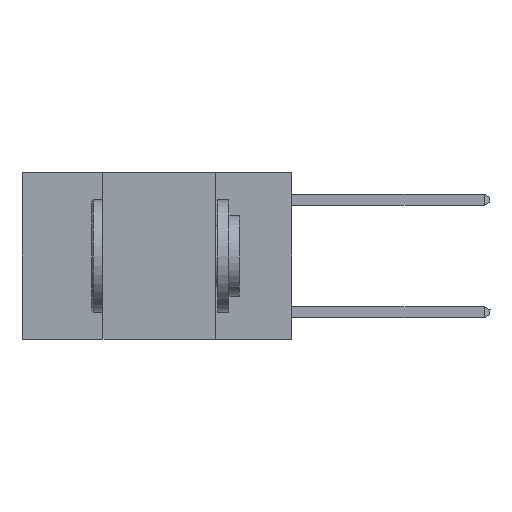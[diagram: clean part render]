
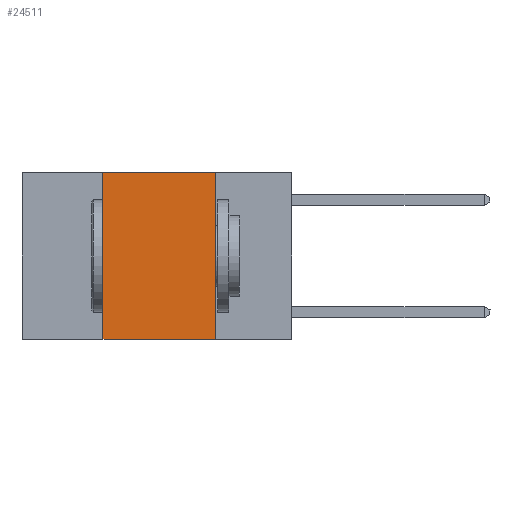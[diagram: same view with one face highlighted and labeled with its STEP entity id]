
A CAD part, left-side view. The second image highlights one B-rep face of the part: STEP entity #24511.
In plain terms, the highlighted planar face has unit normal (-1, 0, 0).
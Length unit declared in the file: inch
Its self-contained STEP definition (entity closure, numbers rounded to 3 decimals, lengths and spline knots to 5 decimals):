
#181 = DIRECTION ( 'NONE',  ( 0., -1., 0. ) ) ;
#733 = ORIENTED_EDGE ( 'NONE', *, *, #6501, .T. ) ;
#1856 = VERTEX_POINT ( 'NONE', #21726 ) ;
#4850 = VERTEX_POINT ( 'NONE', #27027 ) ;
#6138 = DIRECTION ( 'NONE',  ( 0., -1., 0. ) ) ;
#6285 = DIRECTION ( 'NONE',  ( 0., 0., 1. ) ) ;
#6501 = EDGE_CURVE ( 'NONE', #29805, #9033, #10581, .T. ) ;
#7620 = AXIS2_PLACEMENT_3D ( 'NONE', #12785, #10416, #27014 ) ;
#9033 = VERTEX_POINT ( 'NONE', #15039 ) ;
#9204 = VECTOR ( 'NONE', #28720, 39.37008 ) ;
#9432 = VECTOR ( 'NONE', #6285, 39.37008 ) ;
#10416 = DIRECTION ( 'NONE',  ( 1., 0., 0. ) ) ;
#10581 = LINE ( 'NONE', #18218, #16309 ) ;
#12785 = CARTESIAN_POINT ( 'NONE',  ( 0., 0.6, 0. ) ) ;
#13397 = EDGE_CURVE ( 'NONE', #4850, #1856, #19435, .T. ) ;
#13640 = LINE ( 'NONE', #18453, #9432 ) ;
#14961 = CARTESIAN_POINT ( 'NONE',  ( 0., 0.6, 0. ) ) ;
#15039 = CARTESIAN_POINT ( 'NONE',  ( 0., 0.17, -0.37 ) ) ;
#16309 = VECTOR ( 'NONE', #6138, 39.37008 ) ;
#16620 = EDGE_CURVE ( 'NONE', #29805, #4850, #13640, .T. ) ;
#16905 = ORIENTED_EDGE ( 'NONE', *, *, #21106, .F. ) ;
#18218 = CARTESIAN_POINT ( 'NONE',  ( 0., 0.6, -0.37 ) ) ;
#18453 = CARTESIAN_POINT ( 'NONE',  ( 0., 0.42, 0. ) ) ;
#18717 = CARTESIAN_POINT ( 'NONE',  ( 0., 0.42, -0.37 ) ) ;
#19435 = LINE ( 'NONE', #14961, #29465 ) ;
#20021 = PLANE ( 'NONE',  #7620 ) ;
#20223 = ORIENTED_EDGE ( 'NONE', *, *, #16620, .F. ) ;
#20968 = ORIENTED_EDGE ( 'NONE', *, *, #13397, .F. ) ;
#21106 = EDGE_CURVE ( 'NONE', #1856, #9033, #28140, .T. ) ;
#21726 = CARTESIAN_POINT ( 'NONE',  ( 0., 0.17, 0. ) ) ;
#24511 = ADVANCED_FACE ( 'NONE', ( #26876 ), #20021, .F. ) ;
#24699 = EDGE_LOOP ( 'NONE', ( #16905, #20968, #20223, #733 ) ) ;
#26472 = CARTESIAN_POINT ( 'NONE',  ( 0., 0.17, 0. ) ) ;
#26876 = FACE_OUTER_BOUND ( 'NONE', #24699, .T. ) ;
#27014 = DIRECTION ( 'NONE',  ( 0., 0., -1. ) ) ;
#27027 = CARTESIAN_POINT ( 'NONE',  ( 0., 0.42, 0. ) ) ;
#28140 = LINE ( 'NONE', #26472, #9204 ) ;
#28720 = DIRECTION ( 'NONE',  ( 0., 0., -1. ) ) ;
#29465 = VECTOR ( 'NONE', #181, 39.37008 ) ;
#29805 = VERTEX_POINT ( 'NONE', #18717 ) ;
